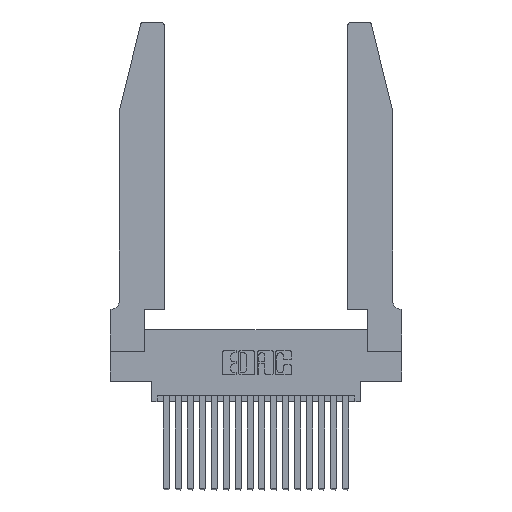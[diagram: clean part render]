
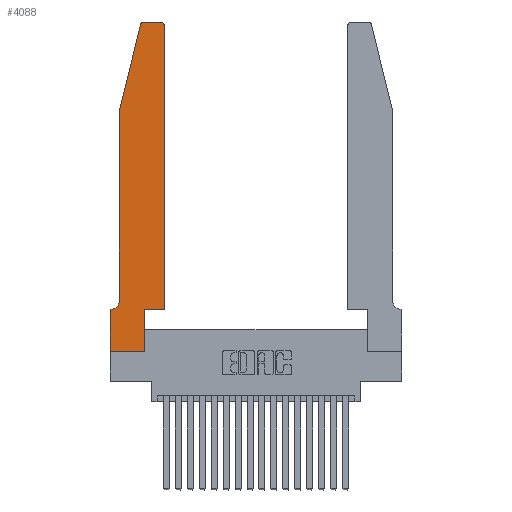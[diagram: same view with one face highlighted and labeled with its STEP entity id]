
A CAD part, top view. The second image highlights one B-rep face of the part: STEP entity #4088.
In plain terms, the highlighted planar face has unit normal (0, 0, 1).
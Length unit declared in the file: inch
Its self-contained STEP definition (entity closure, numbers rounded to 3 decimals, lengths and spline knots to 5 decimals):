
#30 = LINE ( 'NONE', #4809, #16827 ) ;
#86 = ORIENTED_EDGE ( 'NONE', *, *, #1147, .T. ) ;
#368 = CIRCLE ( 'NONE', #11937, 0.03 ) ;
#388 = VECTOR ( 'NONE', #12126, 39.37008 ) ;
#408 = VECTOR ( 'NONE', #8705, 39.37008 ) ;
#453 = EDGE_LOOP ( 'NONE', ( #6955, #19508, #7480, #19980, #16880, #86, #17377, #9534, #13729, #5662, #14243, #10520 ) ) ;
#570 = VECTOR ( 'NONE', #17214, 39.37008 ) ;
#635 = DIRECTION ( 'NONE',  ( 1., 0., 0. ) ) ;
#1147 = EDGE_CURVE ( 'NONE', #3968, #6060, #13023, .T. ) ;
#1295 = CARTESIAN_POINT ( 'NONE',  ( 0.284, 2.72, 0.37 ) ) ;
#1871 = CARTESIAN_POINT ( 'NONE',  ( 0.2605, 2.75, 0.37 ) ) ;
#2059 = CARTESIAN_POINT ( 'NONE',  ( 0.2865, 0.35, 0.37 ) ) ;
#2724 = CARTESIAN_POINT ( 'NONE',  ( 0.25487, 2.72718, 0.37 ) ) ;
#2887 = VERTEX_POINT ( 'NONE', #2724 ) ;
#3020 = DIRECTION ( 'NONE',  ( 1., 0., 0. ) ) ;
#3132 = DIRECTION ( 'NONE',  ( 1., 0., 0. ) ) ;
#3299 = CIRCLE ( 'NONE', #6498, 0.03 ) ;
#3364 = EDGE_CURVE ( 'NONE', #3391, #6499, #17303, .T. ) ;
#3391 = VERTEX_POINT ( 'NONE', #7348 ) ;
#3721 = EDGE_CURVE ( 'NONE', #5888, #7467, #30, .T. ) ;
#3765 = AXIS2_PLACEMENT_3D ( 'NONE', #16796, #10584, #635 ) ;
#3857 = VERTEX_POINT ( 'NONE', #16263 ) ;
#3968 = VERTEX_POINT ( 'NONE', #6967 ) ;
#4088 = ADVANCED_FACE ( 'NONE', ( #10459 ), #19866, .T. ) ;
#4144 = EDGE_CURVE ( 'NONE', #7467, #4639, #5068, .T. ) ;
#4639 = VERTEX_POINT ( 'NONE', #16718 ) ;
#4809 = CARTESIAN_POINT ( 'NONE',  ( 0.4505, 0.35, 0.37 ) ) ;
#4869 = VECTOR ( 'NONE', #11758, 39.37008 ) ;
#4923 = LINE ( 'NONE', #7059, #408 ) ;
#5055 = DIRECTION ( 'NONE',  ( 0., 1., 0. ) ) ;
#5068 = LINE ( 'NONE', #14112, #570 ) ;
#5662 = ORIENTED_EDGE ( 'NONE', *, *, #3721, .T. ) ;
#5888 = VERTEX_POINT ( 'NONE', #2059 ) ;
#6060 = VERTEX_POINT ( 'NONE', #15595 ) ;
#6268 = EDGE_CURVE ( 'NONE', #11711, #13608, #9257, .T. ) ;
#6498 = AXIS2_PLACEMENT_3D ( 'NONE', #17291, #7841, #18819 ) ;
#6499 = VERTEX_POINT ( 'NONE', #16974 ) ;
#6955 = ORIENTED_EDGE ( 'NONE', *, *, #6268, .T. ) ;
#6967 = CARTESIAN_POINT ( 'NONE',  ( 0.0055, 0.35, 0.37 ) ) ;
#7059 = CARTESIAN_POINT ( 'NONE',  ( 0.0755, 2., 0.37 ) ) ;
#7348 = CARTESIAN_POINT ( 'NONE',  ( 0., 0., 0.37 ) ) ;
#7354 = CIRCLE ( 'NONE', #7932, 0.07 ) ;
#7467 = VERTEX_POINT ( 'NONE', #11646 ) ;
#7480 = ORIENTED_EDGE ( 'NONE', *, *, #8191, .T. ) ;
#7565 = CARTESIAN_POINT ( 'NONE',  ( 0., 0., 0.37 ) ) ;
#7824 = VECTOR ( 'NONE', #5055, 39.37008 ) ;
#7841 = DIRECTION ( 'NONE',  ( 0., 0., 1. ) ) ;
#7932 = AXIS2_PLACEMENT_3D ( 'NONE', #9578, #20418, #11174 ) ;
#8191 = EDGE_CURVE ( 'NONE', #2887, #13499, #18467, .T. ) ;
#8705 = DIRECTION ( 'NONE',  ( 0., -1., 0. ) ) ;
#9257 = LINE ( 'NONE', #1871, #4869 ) ;
#9534 = ORIENTED_EDGE ( 'NONE', *, *, #3364, .T. ) ;
#9578 = CARTESIAN_POINT ( 'NONE',  ( 0.0055, 0.42, 0.37 ) ) ;
#9923 = EDGE_CURVE ( 'NONE', #6499, #5888, #16223, .T. ) ;
#10174 = VECTOR ( 'NONE', #16848, 39.37008 ) ;
#10459 = FACE_OUTER_BOUND ( 'NONE', #453, .T. ) ;
#10520 = ORIENTED_EDGE ( 'NONE', *, *, #12329, .T. ) ;
#10584 = DIRECTION ( 'NONE',  ( 0., 0., 1. ) ) ;
#10629 = VECTOR ( 'NONE', #18630, 39.37008 ) ;
#11174 = DIRECTION ( 'NONE',  ( -1., 0., 0. ) ) ;
#11178 = CARTESIAN_POINT ( 'NONE',  ( 0.0755, 2., 0.37 ) ) ;
#11456 = CARTESIAN_POINT ( 'NONE',  ( 0.284, 2.75, 0.37 ) ) ;
#11646 = CARTESIAN_POINT ( 'NONE',  ( 0.4505, 0.35, 0.37 ) ) ;
#11711 = VERTEX_POINT ( 'NONE', #13134 ) ;
#11758 = DIRECTION ( 'NONE',  ( -1., 0., 0. ) ) ;
#11937 = AXIS2_PLACEMENT_3D ( 'NONE', #1295, #12805, #3020 ) ;
#12126 = DIRECTION ( 'NONE',  ( -1., 0., 0. ) ) ;
#12152 = DIRECTION ( 'NONE',  ( 1., 0., 0. ) ) ;
#12154 = CARTESIAN_POINT ( 'NONE',  ( 0.0755, 0.35, 0.37 ) ) ;
#12329 = EDGE_CURVE ( 'NONE', #4639, #11711, #3299, .T. ) ;
#12805 = DIRECTION ( 'NONE',  ( 0., 0., 1. ) ) ;
#13023 = LINE ( 'NONE', #12154, #388 ) ;
#13134 = CARTESIAN_POINT ( 'NONE',  ( 0.4205, 2.75, 0.37 ) ) ;
#13167 = VECTOR ( 'NONE', #12152, 39.37008 ) ;
#13499 = VERTEX_POINT ( 'NONE', #11178 ) ;
#13608 = VERTEX_POINT ( 'NONE', #11456 ) ;
#13729 = ORIENTED_EDGE ( 'NONE', *, *, #9923, .T. ) ;
#14112 = CARTESIAN_POINT ( 'NONE',  ( 0.4505, 0.35, 0.37 ) ) ;
#14243 = ORIENTED_EDGE ( 'NONE', *, *, #4144, .T. ) ;
#14821 = LINE ( 'NONE', #7565, #10629 ) ;
#15249 = CARTESIAN_POINT ( 'NONE',  ( 0.0755, 2., 0.37 ) ) ;
#15456 = EDGE_CURVE ( 'NONE', #3857, #3968, #7354, .T. ) ;
#15595 = CARTESIAN_POINT ( 'NONE',  ( 0., 0.35, 0.37 ) ) ;
#15848 = EDGE_CURVE ( 'NONE', #6060, #3391, #14821, .T. ) ;
#16223 = LINE ( 'NONE', #16247, #7824 ) ;
#16247 = CARTESIAN_POINT ( 'NONE',  ( 0.2865, 0.35, 0.37 ) ) ;
#16263 = CARTESIAN_POINT ( 'NONE',  ( 0.0755, 0.42, 0.37 ) ) ;
#16718 = CARTESIAN_POINT ( 'NONE',  ( 0.4505, 2.72, 0.37 ) ) ;
#16796 = CARTESIAN_POINT ( 'NONE',  ( 0., 0.35, 0.37 ) ) ;
#16827 = VECTOR ( 'NONE', #3132, 39.37008 ) ;
#16848 = DIRECTION ( 'NONE',  ( -0.239, -0.971, 0. ) ) ;
#16880 = ORIENTED_EDGE ( 'NONE', *, *, #15456, .T. ) ;
#16974 = CARTESIAN_POINT ( 'NONE',  ( 0.2865, 0., 0.37 ) ) ;
#17214 = DIRECTION ( 'NONE',  ( 0., 1., 0. ) ) ;
#17291 = CARTESIAN_POINT ( 'NONE',  ( 0.4205, 2.72, 0.37 ) ) ;
#17303 = LINE ( 'NONE', #18309, #13167 ) ;
#17377 = ORIENTED_EDGE ( 'NONE', *, *, #15848, .T. ) ;
#17572 = EDGE_CURVE ( 'NONE', #13499, #3857, #4923, .T. ) ;
#18309 = CARTESIAN_POINT ( 'NONE',  ( 0., 0., 0.37 ) ) ;
#18467 = LINE ( 'NONE', #15249, #10174 ) ;
#18536 = EDGE_CURVE ( 'NONE', #13608, #2887, #368, .T. ) ;
#18630 = DIRECTION ( 'NONE',  ( 0., -1., 0. ) ) ;
#18819 = DIRECTION ( 'NONE',  ( 1., 0., 0. ) ) ;
#19508 = ORIENTED_EDGE ( 'NONE', *, *, #18536, .T. ) ;
#19866 = PLANE ( 'NONE',  #3765 ) ;
#19980 = ORIENTED_EDGE ( 'NONE', *, *, #17572, .T. ) ;
#20418 = DIRECTION ( 'NONE',  ( 0., 0., -1. ) ) ;
